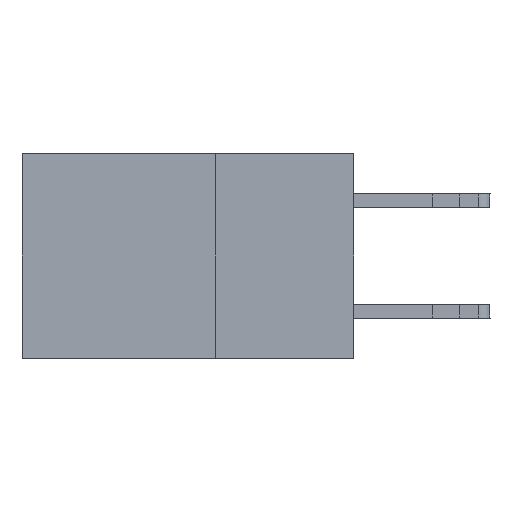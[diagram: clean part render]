
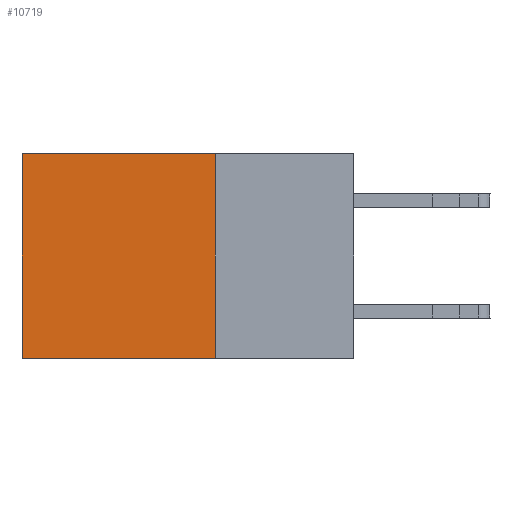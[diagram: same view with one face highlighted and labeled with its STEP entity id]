
A CAD part, left-side view. The second image highlights one B-rep face of the part: STEP entity #10719.
In plain terms, the highlighted planar face has unit normal (-1, 0, 0).
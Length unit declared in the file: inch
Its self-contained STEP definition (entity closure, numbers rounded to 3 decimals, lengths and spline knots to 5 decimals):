
#60 = VERTEX_POINT ( 'NONE', #30438 ) ;
#78 = LINE ( 'NONE', #19687, #5134 ) ;
#853 = CARTESIAN_POINT ( 'NONE',  ( 0.2875, 0.6, -0.37 ) ) ;
#4035 = CARTESIAN_POINT ( 'NONE',  ( 0.2875, 0.25, 0. ) ) ;
#5134 = VECTOR ( 'NONE', #24811, 39.37008 ) ;
#5264 = VECTOR ( 'NONE', #32452, 39.37008 ) ;
#7922 = DIRECTION ( 'NONE',  ( 0., 0., -1. ) ) ;
#8365 = VECTOR ( 'NONE', #23624, 39.37008 ) ;
#9737 = EDGE_LOOP ( 'NONE', ( #18125, #21407, #19683, #15674 ) ) ;
#9847 = PLANE ( 'NONE',  #29406 ) ;
#10649 = CARTESIAN_POINT ( 'NONE',  ( 0.2875, 0.6, 0. ) ) ;
#10719 = ADVANCED_FACE ( 'NONE', ( #20923 ), #9847, .F. ) ;
#11346 = EDGE_CURVE ( 'NONE', #28095, #17703, #19354, .T. ) ;
#14074 = VERTEX_POINT ( 'NONE', #27373 ) ;
#15674 = ORIENTED_EDGE ( 'NONE', *, *, #22951, .T. ) ;
#16229 = CARTESIAN_POINT ( 'NONE',  ( 0.2875, 0.25, 0. ) ) ;
#17201 = VECTOR ( 'NONE', #7922, 39.37008 ) ;
#17483 = DIRECTION ( 'NONE',  ( 0., 0., -1. ) ) ;
#17703 = VERTEX_POINT ( 'NONE', #853 ) ;
#18125 = ORIENTED_EDGE ( 'NONE', *, *, #11346, .T. ) ;
#18459 = EDGE_CURVE ( 'NONE', #14074, #60, #30083, .T. ) ;
#19354 = LINE ( 'NONE', #10649, #17201 ) ;
#19683 = ORIENTED_EDGE ( 'NONE', *, *, #18459, .F. ) ;
#19687 = CARTESIAN_POINT ( 'NONE',  ( 0.2875, 0.25, -0.37 ) ) ;
#20516 = CARTESIAN_POINT ( 'NONE',  ( 0.2875, 0.25, 0. ) ) ;
#20923 = FACE_OUTER_BOUND ( 'NONE', #9737, .T. ) ;
#21407 = ORIENTED_EDGE ( 'NONE', *, *, #29866, .F. ) ;
#22951 = EDGE_CURVE ( 'NONE', #14074, #28095, #29272, .T. ) ;
#23624 = DIRECTION ( 'NONE',  ( 0., 1., 0. ) ) ;
#24078 = CARTESIAN_POINT ( 'NONE',  ( 0.2875, 0.6, 0. ) ) ;
#24811 = DIRECTION ( 'NONE',  ( 0., 1., 0. ) ) ;
#27373 = CARTESIAN_POINT ( 'NONE',  ( 0.2875, 0.25, 0. ) ) ;
#28095 = VERTEX_POINT ( 'NONE', #24078 ) ;
#29272 = LINE ( 'NONE', #20516, #8365 ) ;
#29406 = AXIS2_PLACEMENT_3D ( 'NONE', #4035, #34059, #17483 ) ;
#29866 = EDGE_CURVE ( 'NONE', #60, #17703, #78, .T. ) ;
#30083 = LINE ( 'NONE', #16229, #5264 ) ;
#30438 = CARTESIAN_POINT ( 'NONE',  ( 0.2875, 0.25, -0.37 ) ) ;
#32452 = DIRECTION ( 'NONE',  ( 0., 0., -1. ) ) ;
#34059 = DIRECTION ( 'NONE',  ( 1., 0., 0. ) ) ;
